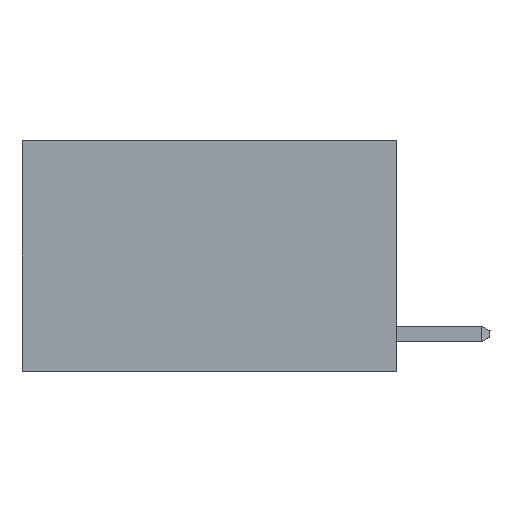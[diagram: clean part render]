
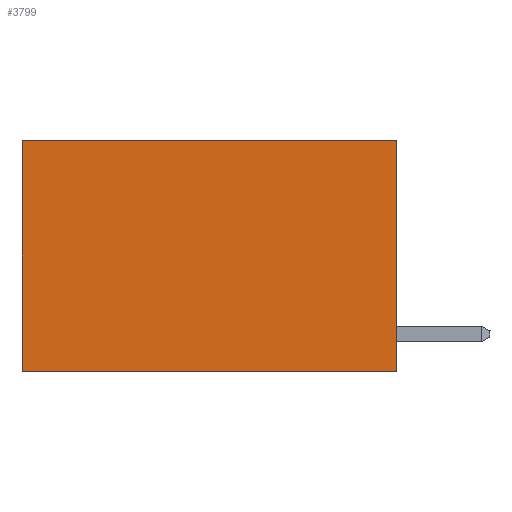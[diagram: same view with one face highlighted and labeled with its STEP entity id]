
A CAD part, left-side view. The second image highlights one B-rep face of the part: STEP entity #3799.
In plain terms, the highlighted planar face has unit normal (-1, 0, 0).
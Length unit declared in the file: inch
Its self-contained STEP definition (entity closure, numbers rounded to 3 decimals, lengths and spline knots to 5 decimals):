
#68 = ORIENTED_EDGE ( 'NONE', *, *, #7872, .F. ) ;
#157 = LINE ( 'NONE', #5816, #8542 ) ;
#196 = ORIENTED_EDGE ( 'NONE', *, *, #317, .T. ) ;
#317 = EDGE_CURVE ( 'NONE', #1039, #5944, #880, .T. ) ;
#811 = VECTOR ( 'NONE', #7438, 39.37008 ) ;
#861 = ORIENTED_EDGE ( 'NONE', *, *, #8553, .F. ) ;
#880 = LINE ( 'NONE', #6147, #3979 ) ;
#921 = FACE_OUTER_BOUND ( 'NONE', #9241, .T. ) ;
#1039 = VERTEX_POINT ( 'NONE', #5239 ) ;
#1769 = CARTESIAN_POINT ( 'NONE',  ( 0.2625, 0., -0.37 ) ) ;
#1869 = LINE ( 'NONE', #6739, #6046 ) ;
#1892 = DIRECTION ( 'NONE',  ( 0., 1., 0. ) ) ;
#2150 = DIRECTION ( 'NONE',  ( 0., 0., -1. ) ) ;
#2398 = VERTEX_POINT ( 'NONE', #6883 ) ;
#2618 = DIRECTION ( 'NONE',  ( 1., 0., 0. ) ) ;
#2783 = AXIS2_PLACEMENT_3D ( 'NONE', #6965, #2618, #6877 ) ;
#3799 = ADVANCED_FACE ( 'NONE', ( #921 ), #8340, .F. ) ;
#3979 = VECTOR ( 'NONE', #1892, 39.37008 ) ;
#4796 = CARTESIAN_POINT ( 'NONE',  ( 0.2625, 0., -0.37 ) ) ;
#5239 = CARTESIAN_POINT ( 'NONE',  ( 0.2625, 0., 0. ) ) ;
#5452 = EDGE_CURVE ( 'NONE', #5944, #2398, #1869, .T. ) ;
#5816 = CARTESIAN_POINT ( 'NONE',  ( 0.2625, 0., 0. ) ) ;
#5885 = LINE ( 'NONE', #1769, #811 ) ;
#5944 = VERTEX_POINT ( 'NONE', #7469 ) ;
#6046 = VECTOR ( 'NONE', #8175, 39.37008 ) ;
#6147 = CARTESIAN_POINT ( 'NONE',  ( 0.2625, 0., 0. ) ) ;
#6739 = CARTESIAN_POINT ( 'NONE',  ( 0.2625, 0.6, 0. ) ) ;
#6877 = DIRECTION ( 'NONE',  ( 0., 0., -1. ) ) ;
#6883 = CARTESIAN_POINT ( 'NONE',  ( 0.2625, 0.6, -0.37 ) ) ;
#6965 = CARTESIAN_POINT ( 'NONE',  ( 0.2625, 0., 0. ) ) ;
#7438 = DIRECTION ( 'NONE',  ( 0., 1., 0. ) ) ;
#7469 = CARTESIAN_POINT ( 'NONE',  ( 0.2625, 0.6, 0. ) ) ;
#7872 = EDGE_CURVE ( 'NONE', #8666, #2398, #5885, .T. ) ;
#8175 = DIRECTION ( 'NONE',  ( 0., 0., -1. ) ) ;
#8340 = PLANE ( 'NONE',  #2783 ) ;
#8542 = VECTOR ( 'NONE', #2150, 39.37008 ) ;
#8553 = EDGE_CURVE ( 'NONE', #1039, #8666, #157, .T. ) ;
#8666 = VERTEX_POINT ( 'NONE', #4796 ) ;
#8722 = ORIENTED_EDGE ( 'NONE', *, *, #5452, .T. ) ;
#9241 = EDGE_LOOP ( 'NONE', ( #8722, #68, #861, #196 ) ) ;
